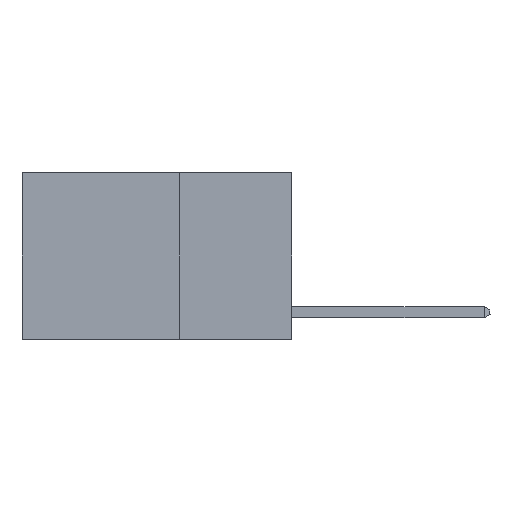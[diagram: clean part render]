
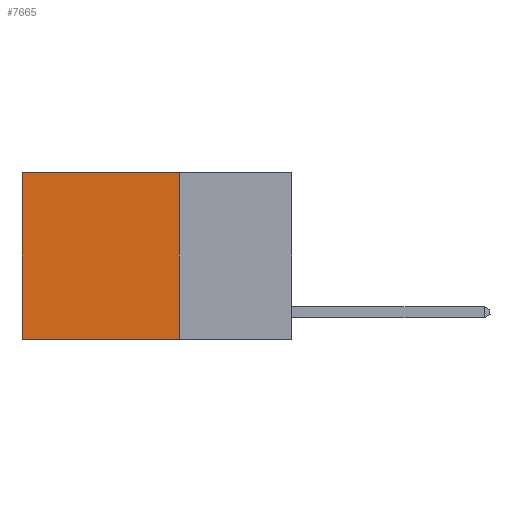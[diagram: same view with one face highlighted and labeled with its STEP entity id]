
A CAD part, left-side view. The second image highlights one B-rep face of the part: STEP entity #7665.
In plain terms, the highlighted planar face has unit normal (-1, 0, 0).
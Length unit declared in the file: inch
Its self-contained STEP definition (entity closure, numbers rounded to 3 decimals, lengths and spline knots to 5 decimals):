
#366 = ORIENTED_EDGE ( 'NONE', *, *, #22435, .F. ) ;
#1500 = EDGE_CURVE ( 'NONE', #10939, #4632, #18798, .T. ) ;
#1742 = AXIS2_PLACEMENT_3D ( 'NONE', #15456, #3286, #2818 ) ;
#2309 = CARTESIAN_POINT ( 'NONE',  ( 0.2625, 0.25, -0.37 ) ) ;
#2407 = DIRECTION ( 'NONE',  ( 0., 0., -1. ) ) ;
#2631 = CARTESIAN_POINT ( 'NONE',  ( 0.2625, 0.6, 0. ) ) ;
#2818 = DIRECTION ( 'NONE',  ( 0., 0., -1. ) ) ;
#2861 = CARTESIAN_POINT ( 'NONE',  ( 0.2625, 0.25, -0.37 ) ) ;
#3046 = FACE_OUTER_BOUND ( 'NONE', #15626, .T. ) ;
#3286 = DIRECTION ( 'NONE',  ( 1., 0., 0. ) ) ;
#4449 = CARTESIAN_POINT ( 'NONE',  ( 0.2625, 0.6, 0. ) ) ;
#4632 = VERTEX_POINT ( 'NONE', #4449 ) ;
#6983 = VECTOR ( 'NONE', #2407, 39.37008 ) ;
#7665 = ADVANCED_FACE ( 'NONE', ( #3046 ), #11835, .F. ) ;
#8536 = ORIENTED_EDGE ( 'NONE', *, *, #9233, .T. ) ;
#9233 = EDGE_CURVE ( 'NONE', #4632, #9856, #12621, .T. ) ;
#9856 = VERTEX_POINT ( 'NONE', #22428 ) ;
#10029 = DIRECTION ( 'NONE',  ( 0., 1., 0. ) ) ;
#10087 = CARTESIAN_POINT ( 'NONE',  ( 0.2625, 0.25, 0. ) ) ;
#10217 = ORIENTED_EDGE ( 'NONE', *, *, #17761, .F. ) ;
#10414 = CARTESIAN_POINT ( 'NONE',  ( 0.2625, 0.25, 0. ) ) ;
#10939 = VERTEX_POINT ( 'NONE', #10414 ) ;
#11051 = LINE ( 'NONE', #15946, #17215 ) ;
#11835 = PLANE ( 'NONE',  #1742 ) ;
#11998 = LINE ( 'NONE', #2861, #14988 ) ;
#12621 = LINE ( 'NONE', #2631, #6983 ) ;
#14988 = VECTOR ( 'NONE', #10029, 39.37008 ) ;
#15456 = CARTESIAN_POINT ( 'NONE',  ( 0.2625, 0.25, 0. ) ) ;
#15626 = EDGE_LOOP ( 'NONE', ( #8536, #366, #10217, #18932 ) ) ;
#15946 = CARTESIAN_POINT ( 'NONE',  ( 0.2625, 0.25, 0. ) ) ;
#17215 = VECTOR ( 'NONE', #18140, 39.37008 ) ;
#17761 = EDGE_CURVE ( 'NONE', #10939, #20103, #11051, .T. ) ;
#18140 = DIRECTION ( 'NONE',  ( 0., 0., -1. ) ) ;
#18798 = LINE ( 'NONE', #10087, #22037 ) ;
#18932 = ORIENTED_EDGE ( 'NONE', *, *, #1500, .T. ) ;
#19030 = DIRECTION ( 'NONE',  ( 0., 1., 0. ) ) ;
#20103 = VERTEX_POINT ( 'NONE', #2309 ) ;
#22037 = VECTOR ( 'NONE', #19030, 39.37008 ) ;
#22428 = CARTESIAN_POINT ( 'NONE',  ( 0.2625, 0.6, -0.37 ) ) ;
#22435 = EDGE_CURVE ( 'NONE', #20103, #9856, #11998, .T. ) ;
